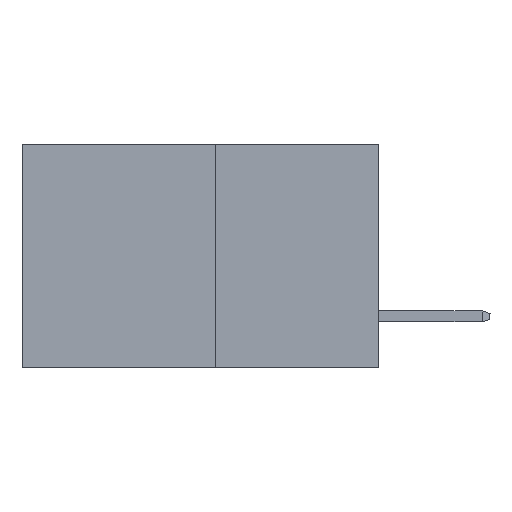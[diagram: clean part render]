
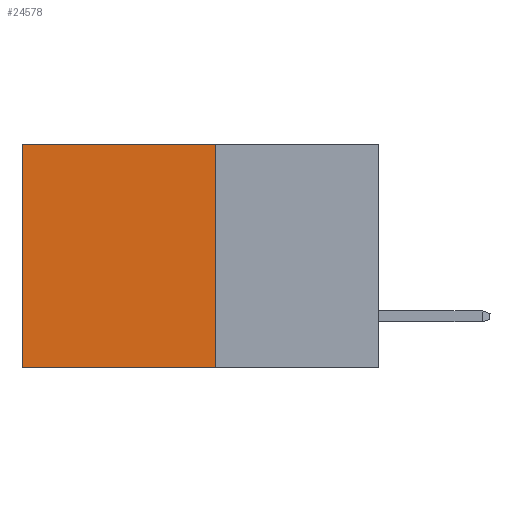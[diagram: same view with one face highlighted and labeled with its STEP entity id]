
A CAD part, left-side view. The second image highlights one B-rep face of the part: STEP entity #24578.
In plain terms, the highlighted planar face has unit normal (-1, 0, 0).
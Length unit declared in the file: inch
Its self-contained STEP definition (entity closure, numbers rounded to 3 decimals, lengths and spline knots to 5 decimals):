
#121 = CARTESIAN_POINT ( 'NONE',  ( 0.277, 0.27, -0.37 ) ) ;
#1285 = CARTESIAN_POINT ( 'NONE',  ( 0.277, 0.59, 0. ) ) ;
#1349 = VECTOR ( 'NONE', #23064, 39.37008 ) ;
#2150 = CARTESIAN_POINT ( 'NONE',  ( 0.277, 0.27, 0. ) ) ;
#2162 = DIRECTION ( 'NONE',  ( 0., 0., -1. ) ) ;
#2452 = VERTEX_POINT ( 'NONE', #2150 ) ;
#5232 = VERTEX_POINT ( 'NONE', #10245 ) ;
#5321 = LINE ( 'NONE', #9462, #22704 ) ;
#6254 = VERTEX_POINT ( 'NONE', #22292 ) ;
#6552 = CARTESIAN_POINT ( 'NONE',  ( 0.277, 0.59, -0.37 ) ) ;
#6639 = ORIENTED_EDGE ( 'NONE', *, *, #8788, .T. ) ;
#6900 = AXIS2_PLACEMENT_3D ( 'NONE', #12831, #14964, #2162 ) ;
#8788 = EDGE_CURVE ( 'NONE', #20180, #5232, #13311, .T. ) ;
#9462 = CARTESIAN_POINT ( 'NONE',  ( 0.277, 0.27, 0. ) ) ;
#10115 = ORIENTED_EDGE ( 'NONE', *, *, #18691, .F. ) ;
#10245 = CARTESIAN_POINT ( 'NONE',  ( 0.277, 0.59, -0.37 ) ) ;
#12738 = LINE ( 'NONE', #20990, #1349 ) ;
#12831 = CARTESIAN_POINT ( 'NONE',  ( 0.277, 0.27, -0.37 ) ) ;
#12832 = ORIENTED_EDGE ( 'NONE', *, *, #23994, .F. ) ;
#13311 = LINE ( 'NONE', #6552, #23638 ) ;
#13706 = FACE_OUTER_BOUND ( 'NONE', #20903, .T. ) ;
#14964 = DIRECTION ( 'NONE',  ( 1., 0., 0. ) ) ;
#15735 = EDGE_CURVE ( 'NONE', #2452, #20180, #5321, .T. ) ;
#18691 = EDGE_CURVE ( 'NONE', #6254, #5232, #19669, .T. ) ;
#19669 = LINE ( 'NONE', #121, #24505 ) ;
#20180 = VERTEX_POINT ( 'NONE', #1285 ) ;
#20903 = EDGE_LOOP ( 'NONE', ( #6639, #10115, #12832, #21857 ) ) ;
#20990 = CARTESIAN_POINT ( 'NONE',  ( 0.277, 0.27, -0.37 ) ) ;
#21180 = DIRECTION ( 'NONE',  ( 0., 1., 0. ) ) ;
#21219 = DIRECTION ( 'NONE',  ( 0., 0., -1. ) ) ;
#21857 = ORIENTED_EDGE ( 'NONE', *, *, #15735, .T. ) ;
#22292 = CARTESIAN_POINT ( 'NONE',  ( 0.277, 0.27, -0.37 ) ) ;
#22704 = VECTOR ( 'NONE', #26043, 39.37008 ) ;
#23064 = DIRECTION ( 'NONE',  ( 0., 0., -1. ) ) ;
#23638 = VECTOR ( 'NONE', #21219, 39.37008 ) ;
#23994 = EDGE_CURVE ( 'NONE', #2452, #6254, #12738, .T. ) ;
#24505 = VECTOR ( 'NONE', #21180, 39.37008 ) ;
#24578 = ADVANCED_FACE ( 'NONE', ( #13706 ), #25190, .F. ) ;
#25190 = PLANE ( 'NONE',  #6900 ) ;
#26043 = DIRECTION ( 'NONE',  ( 0., 1., 0. ) ) ;
